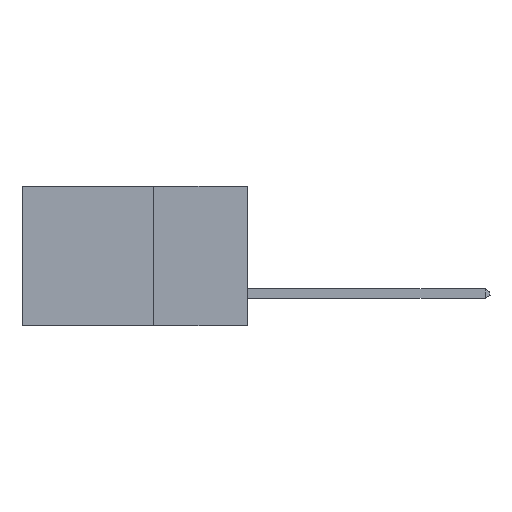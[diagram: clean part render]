
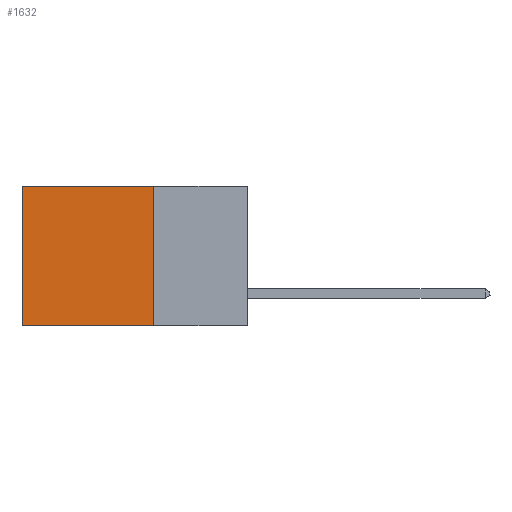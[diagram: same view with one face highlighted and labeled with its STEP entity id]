
A CAD part, left-side view. The second image highlights one B-rep face of the part: STEP entity #1632.
In plain terms, the highlighted planar face has unit normal (-1, 0, 0).
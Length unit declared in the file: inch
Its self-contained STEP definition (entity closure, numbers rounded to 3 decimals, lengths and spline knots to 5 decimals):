
#16 = CARTESIAN_POINT ( 'NONE',  ( 0.298, 0.6, -0.37 ) ) ;
#55 = VERTEX_POINT ( 'NONE', #4880 ) ;
#472 = LINE ( 'NONE', #9288, #9337 ) ;
#1347 = CARTESIAN_POINT ( 'NONE',  ( 0.298, 0.25, -0.37 ) ) ;
#1632 = ADVANCED_FACE ( 'NONE', ( #5921 ), #11619, .F. ) ;
#1868 = DIRECTION ( 'NONE',  ( 0., 0., -1. ) ) ;
#2665 = CARTESIAN_POINT ( 'NONE',  ( 0.298, 0.6, 0. ) ) ;
#3399 = VECTOR ( 'NONE', #16703, 39.37008 ) ;
#3730 = DIRECTION ( 'NONE',  ( 0., 1., 0. ) ) ;
#3778 = EDGE_CURVE ( 'NONE', #12902, #55, #10307, .T. ) ;
#4089 = EDGE_CURVE ( 'NONE', #12902, #15168, #13148, .T. ) ;
#4880 = CARTESIAN_POINT ( 'NONE',  ( 0.298, 0.25, -0.37 ) ) ;
#5412 = ORIENTED_EDGE ( 'NONE', *, *, #3778, .F. ) ;
#5813 = DIRECTION ( 'NONE',  ( 0., 0., -1. ) ) ;
#5903 = CARTESIAN_POINT ( 'NONE',  ( 0.298, 0.25, 0. ) ) ;
#5921 = FACE_OUTER_BOUND ( 'NONE', #14347, .T. ) ;
#6155 = CARTESIAN_POINT ( 'NONE',  ( 0.298, 0.25, 0. ) ) ;
#6568 = CARTESIAN_POINT ( 'NONE',  ( 0.298, 0.25, 0. ) ) ;
#6973 = VECTOR ( 'NONE', #3730, 39.37008 ) ;
#8547 = DIRECTION ( 'NONE',  ( 1., 0., 0. ) ) ;
#9204 = AXIS2_PLACEMENT_3D ( 'NONE', #17114, #8547, #5813 ) ;
#9288 = CARTESIAN_POINT ( 'NONE',  ( 0.298, 0.6, 0. ) ) ;
#9337 = VECTOR ( 'NONE', #12241, 39.37008 ) ;
#9429 = VECTOR ( 'NONE', #1868, 39.37008 ) ;
#10307 = LINE ( 'NONE', #6155, #9429 ) ;
#10609 = EDGE_CURVE ( 'NONE', #55, #13170, #13122, .T. ) ;
#11271 = ORIENTED_EDGE ( 'NONE', *, *, #10609, .F. ) ;
#11619 = PLANE ( 'NONE',  #9204 ) ;
#12241 = DIRECTION ( 'NONE',  ( 0., 0., -1. ) ) ;
#12726 = ORIENTED_EDGE ( 'NONE', *, *, #4089, .T. ) ;
#12902 = VERTEX_POINT ( 'NONE', #5903 ) ;
#13122 = LINE ( 'NONE', #1347, #3399 ) ;
#13148 = LINE ( 'NONE', #6568, #6973 ) ;
#13170 = VERTEX_POINT ( 'NONE', #16 ) ;
#14347 = EDGE_LOOP ( 'NONE', ( #15264, #11271, #5412, #12726 ) ) ;
#15168 = VERTEX_POINT ( 'NONE', #2665 ) ;
#15264 = ORIENTED_EDGE ( 'NONE', *, *, #17787, .T. ) ;
#16703 = DIRECTION ( 'NONE',  ( 0., 1., 0. ) ) ;
#17114 = CARTESIAN_POINT ( 'NONE',  ( 0.298, 0.25, 0. ) ) ;
#17787 = EDGE_CURVE ( 'NONE', #15168, #13170, #472, .T. ) ;
